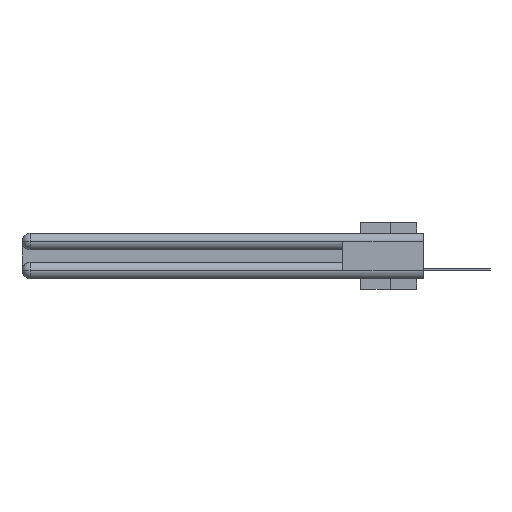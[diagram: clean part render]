
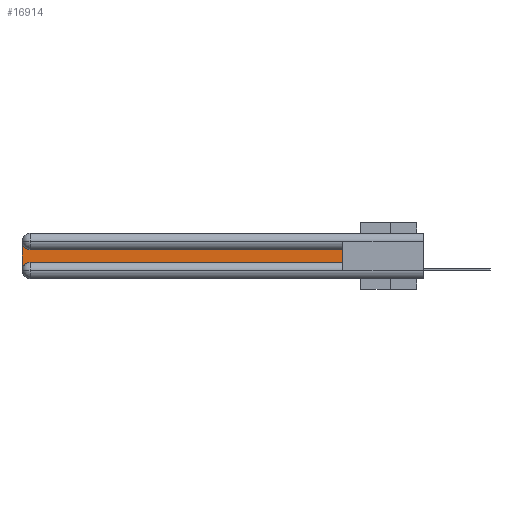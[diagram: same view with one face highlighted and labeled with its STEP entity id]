
A CAD part, left-side view. The second image highlights one B-rep face of the part: STEP entity #16914.
In plain terms, the highlighted planar face has unit normal (-1, 0, 0).
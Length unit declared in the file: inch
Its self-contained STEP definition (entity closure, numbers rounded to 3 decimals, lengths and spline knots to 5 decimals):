
#818 = EDGE_CURVE ( 'NONE', #1126, #23905, #9841, .T. ) ;
#1053 = CARTESIAN_POINT ( 'NONE',  ( 0.075, 0.6, -0.1225 ) ) ;
#1126 = VERTEX_POINT ( 'NONE', #13728 ) ;
#1685 = DIRECTION ( 'NONE',  ( 0., 0., -1. ) ) ;
#2050 = VERTEX_POINT ( 'NONE', #1053 ) ;
#2585 = ORIENTED_EDGE ( 'NONE', *, *, #6948, .T. ) ;
#2616 = CARTESIAN_POINT ( 'NONE',  ( 0.075, 0.6, -0.1225 ) ) ;
#3277 = VECTOR ( 'NONE', #23256, 39.37008 ) ;
#4079 = CARTESIAN_POINT ( 'NONE',  ( 0.075, 0.6, -0.2175 ) ) ;
#5151 = LINE ( 'NONE', #2616, #3277 ) ;
#5287 = AXIS2_PLACEMENT_3D ( 'NONE', #11995, #21965, #14038 ) ;
#6114 = AXIS2_PLACEMENT_3D ( 'NONE', #7367, #17861, #14994 ) ;
#6948 = EDGE_CURVE ( 'NONE', #13652, #2050, #27291, .T. ) ;
#7367 = CARTESIAN_POINT ( 'NONE',  ( 0.075, 2.94, -0.2775 ) ) ;
#8201 = DIRECTION ( 'NONE',  ( 0., 0., -1. ) ) ;
#9273 = LINE ( 'NONE', #11662, #9396 ) ;
#9334 = DIRECTION ( 'NONE',  ( 0., 0., 1. ) ) ;
#9396 = VECTOR ( 'NONE', #21966, 39.37008 ) ;
#9841 = LINE ( 'NONE', #20155, #12002 ) ;
#10705 = CIRCLE ( 'NONE', #5287, 0.06 ) ;
#11662 = CARTESIAN_POINT ( 'NONE',  ( 0.075, 0.6, -0.2175 ) ) ;
#11995 = CARTESIAN_POINT ( 'NONE',  ( 0.075, 2.94, -0.0625 ) ) ;
#12002 = VECTOR ( 'NONE', #1685, 39.37008 ) ;
#13136 = PLANE ( 'NONE',  #30588 ) ;
#13652 = VERTEX_POINT ( 'NONE', #18152 ) ;
#13728 = CARTESIAN_POINT ( 'NONE',  ( 0.075, 3., -0.0625 ) ) ;
#14038 = DIRECTION ( 'NONE',  ( 0., 0., -1. ) ) ;
#14399 = EDGE_CURVE ( 'NONE', #21257, #13652, #9273, .T. ) ;
#14682 = ORIENTED_EDGE ( 'NONE', *, *, #21012, .T. ) ;
#14994 = DIRECTION ( 'NONE',  ( 0., 0., -1. ) ) ;
#16185 = CARTESIAN_POINT ( 'NONE',  ( 0.075, 3., -0.1225 ) ) ;
#16914 = ADVANCED_FACE ( 'NONE', ( #29216 ), #13136, .F. ) ;
#17861 = DIRECTION ( 'NONE',  ( 1., 0., 0. ) ) ;
#18152 = CARTESIAN_POINT ( 'NONE',  ( 0.075, 0.6, -0.2175 ) ) ;
#19533 = ORIENTED_EDGE ( 'NONE', *, *, #818, .T. ) ;
#20141 = CIRCLE ( 'NONE', #6114, 0.06 ) ;
#20155 = CARTESIAN_POINT ( 'NONE',  ( 0.075, 3., -0.2175 ) ) ;
#20966 = ORIENTED_EDGE ( 'NONE', *, *, #14399, .T. ) ;
#21012 = EDGE_CURVE ( 'NONE', #24562, #1126, #10705, .T. ) ;
#21257 = VERTEX_POINT ( 'NONE', #28747 ) ;
#21965 = DIRECTION ( 'NONE',  ( 1., 0., 0. ) ) ;
#21966 = DIRECTION ( 'NONE',  ( 0., -1., 0. ) ) ;
#23256 = DIRECTION ( 'NONE',  ( 0., 1., 0. ) ) ;
#23862 = CARTESIAN_POINT ( 'NONE',  ( 0.075, 2.94, -0.1225 ) ) ;
#23905 = VERTEX_POINT ( 'NONE', #28209 ) ;
#24457 = ORIENTED_EDGE ( 'NONE', *, *, #33401, .T. ) ;
#24562 = VERTEX_POINT ( 'NONE', #23862 ) ;
#26146 = DIRECTION ( 'NONE',  ( 1., 0., 0. ) ) ;
#27291 = LINE ( 'NONE', #4079, #27799 ) ;
#27799 = VECTOR ( 'NONE', #9334, 39.37008 ) ;
#28209 = CARTESIAN_POINT ( 'NONE',  ( 0.075, 3., -0.2775 ) ) ;
#28747 = CARTESIAN_POINT ( 'NONE',  ( 0.075, 2.94, -0.2175 ) ) ;
#29216 = FACE_OUTER_BOUND ( 'NONE', #33092, .T. ) ;
#29938 = EDGE_CURVE ( 'NONE', #2050, #24562, #5151, .T. ) ;
#30434 = ORIENTED_EDGE ( 'NONE', *, *, #29938, .T. ) ;
#30588 = AXIS2_PLACEMENT_3D ( 'NONE', #16185, #26146, #8201 ) ;
#33092 = EDGE_LOOP ( 'NONE', ( #30434, #14682, #19533, #24457, #20966, #2585 ) ) ;
#33401 = EDGE_CURVE ( 'NONE', #23905, #21257, #20141, .T. ) ;
